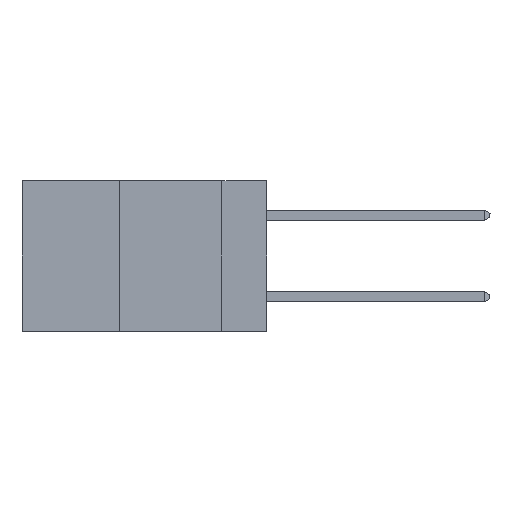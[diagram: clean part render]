
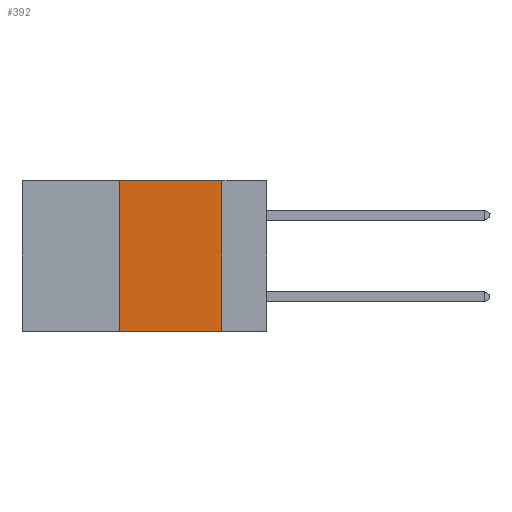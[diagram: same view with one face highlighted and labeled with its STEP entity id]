
A CAD part, left-side view. The second image highlights one B-rep face of the part: STEP entity #392.
In plain terms, the highlighted planar face has unit normal (-1, 0, 0).
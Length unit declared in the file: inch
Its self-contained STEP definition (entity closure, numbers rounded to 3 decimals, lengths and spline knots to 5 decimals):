
#392 = ADVANCED_FACE ( 'NONE', ( #23780 ), #13087, .F. ) ;
#2657 = AXIS2_PLACEMENT_3D ( 'NONE', #23051, #25147, #8874 ) ;
#3169 = VECTOR ( 'NONE', #10531, 39.37008 ) ;
#3188 = VERTEX_POINT ( 'NONE', #13051 ) ;
#3462 = EDGE_CURVE ( 'NONE', #14961, #17113, #15703, .T. ) ;
#3829 = EDGE_CURVE ( 'NONE', #14961, #16490, #12862, .T. ) ;
#3969 = CARTESIAN_POINT ( 'NONE',  ( 0., 0.36, 0. ) ) ;
#4239 = CARTESIAN_POINT ( 'NONE',  ( 0., 0.6, 0. ) ) ;
#7044 = CARTESIAN_POINT ( 'NONE',  ( 0., 0.11, -0.37 ) ) ;
#7856 = DIRECTION ( 'NONE',  ( 0., -1., 0. ) ) ;
#8692 = ORIENTED_EDGE ( 'NONE', *, *, #3829, .F. ) ;
#8874 = DIRECTION ( 'NONE',  ( 0., 0., -1. ) ) ;
#10364 = VECTOR ( 'NONE', #7856, 39.37008 ) ;
#10531 = DIRECTION ( 'NONE',  ( 0., 0., 1. ) ) ;
#10558 = EDGE_CURVE ( 'NONE', #16490, #3188, #12485, .T. ) ;
#10879 = EDGE_CURVE ( 'NONE', #3188, #17113, #25314, .T. ) ;
#11401 = ORIENTED_EDGE ( 'NONE', *, *, #10558, .F. ) ;
#12485 = LINE ( 'NONE', #4239, #22479 ) ;
#12862 = LINE ( 'NONE', #22513, #3169 ) ;
#13051 = CARTESIAN_POINT ( 'NONE',  ( 0., 0.11, 0. ) ) ;
#13087 = PLANE ( 'NONE',  #2657 ) ;
#13895 = CARTESIAN_POINT ( 'NONE',  ( 0., 0.36, -0.37 ) ) ;
#14961 = VERTEX_POINT ( 'NONE', #13895 ) ;
#15099 = CARTESIAN_POINT ( 'NONE',  ( 0., 0.11, 0. ) ) ;
#15698 = ORIENTED_EDGE ( 'NONE', *, *, #3462, .T. ) ;
#15703 = LINE ( 'NONE', #15897, #10364 ) ;
#15897 = CARTESIAN_POINT ( 'NONE',  ( 0., 0.6, -0.37 ) ) ;
#16490 = VERTEX_POINT ( 'NONE', #3969 ) ;
#17113 = VERTEX_POINT ( 'NONE', #7044 ) ;
#17372 = DIRECTION ( 'NONE',  ( 0., 0., -1. ) ) ;
#18750 = VECTOR ( 'NONE', #17372, 39.37008 ) ;
#19157 = ORIENTED_EDGE ( 'NONE', *, *, #10879, .F. ) ;
#22479 = VECTOR ( 'NONE', #24326, 39.37008 ) ;
#22513 = CARTESIAN_POINT ( 'NONE',  ( 0., 0.36, 0. ) ) ;
#23051 = CARTESIAN_POINT ( 'NONE',  ( 0., 0.6, 0. ) ) ;
#23780 = FACE_OUTER_BOUND ( 'NONE', #24651, .T. ) ;
#24326 = DIRECTION ( 'NONE',  ( 0., -1., 0. ) ) ;
#24651 = EDGE_LOOP ( 'NONE', ( #19157, #11401, #8692, #15698 ) ) ;
#25147 = DIRECTION ( 'NONE',  ( 1., 0., 0. ) ) ;
#25314 = LINE ( 'NONE', #15099, #18750 ) ;
